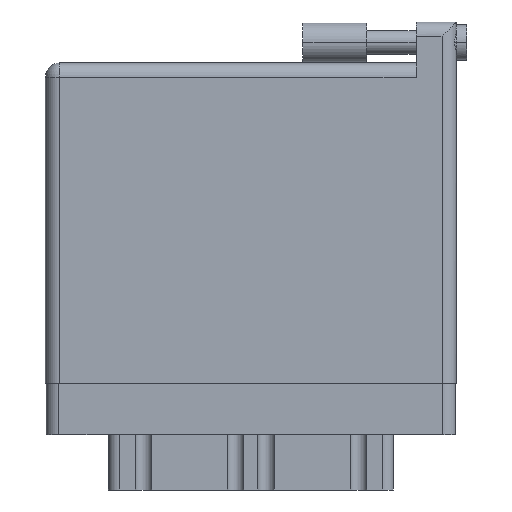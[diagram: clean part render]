
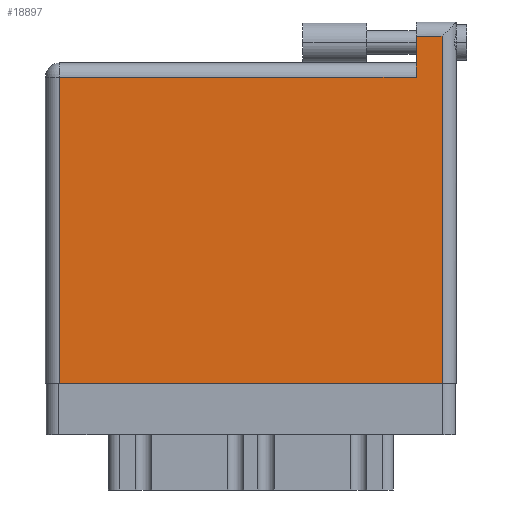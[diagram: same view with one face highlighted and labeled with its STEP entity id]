
A CAD part, front view. The second image highlights one B-rep face of the part: STEP entity #18897.
In plain terms, the highlighted face is planar.
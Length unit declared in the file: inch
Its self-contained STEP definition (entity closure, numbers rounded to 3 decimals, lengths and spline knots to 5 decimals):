
#985 = DIRECTION ( 'NONE',  ( 1., 0., 0. ) ) ;
#2232 = CARTESIAN_POINT ( 'NONE',  ( 0.07, 0., 0. ) ) ;
#2502 = ORIENTED_EDGE ( 'NONE', *, *, #12456, .T. ) ;
#2968 = ORIENTED_EDGE ( 'NONE', *, *, #26892, .T. ) ;
#3290 = FACE_OUTER_BOUND ( 'NONE', #28474, .T. ) ;
#3557 = LINE ( 'NONE', #14199, #27384 ) ;
#4309 = CARTESIAN_POINT ( 'NONE',  ( 0., 1.696, 0. ) ) ;
#5326 = VECTOR ( 'NONE', #9005, 39.37008 ) ;
#5433 = CARTESIAN_POINT ( 'NONE',  ( 1.811, 1.766, 0. ) ) ;
#7760 = VECTOR ( 'NONE', #30245, 39.37008 ) ;
#9005 = DIRECTION ( 'NONE',  ( 0., -1., 0. ) ) ;
#9722 = VECTOR ( 'NONE', #985, 39.37008 ) ;
#9880 = AXIS2_PLACEMENT_3D ( 'NONE', #11156, #13936, #21934 ) ;
#11032 = LINE ( 'NONE', #5433, #19995 ) ;
#11156 = CARTESIAN_POINT ( 'NONE',  ( 0., 1.566, 0. ) ) ;
#11453 = LINE ( 'NONE', #25028, #5326 ) ;
#12249 = VERTEX_POINT ( 'NONE', #2232 ) ;
#12456 = EDGE_CURVE ( 'NONE', #12249, #24019, #30618, .T. ) ;
#12862 = VERTEX_POINT ( 'NONE', #22873 ) ;
#13936 = DIRECTION ( 'NONE',  ( 0., 0., -1. ) ) ;
#14069 = EDGE_CURVE ( 'NONE', #22793, #12862, #11032, .T. ) ;
#14199 = CARTESIAN_POINT ( 'NONE',  ( 1.938, 1.766, 0. ) ) ;
#16367 = ORIENTED_EDGE ( 'NONE', *, *, #14069, .T. ) ;
#17298 = CARTESIAN_POINT ( 'NONE',  ( 0.07, 1.496, 0. ) ) ;
#17603 = EDGE_CURVE ( 'NONE', #21061, #12249, #11453, .T. ) ;
#17937 = CARTESIAN_POINT ( 'NONE',  ( 1.811, 1.696, 0. ) ) ;
#18210 = ORIENTED_EDGE ( 'NONE', *, *, #29429, .T. ) ;
#18897 = ADVANCED_FACE ( 'NONE', ( #3290 ), #29606, .F. ) ;
#19389 = CARTESIAN_POINT ( 'NONE',  ( 1.938, 0., 0. ) ) ;
#19602 = DIRECTION ( 'NONE',  ( 0., 1., 0. ) ) ;
#19995 = VECTOR ( 'NONE', #31580, 39.37008 ) ;
#21061 = VERTEX_POINT ( 'NONE', #17298 ) ;
#21934 = DIRECTION ( 'NONE',  ( -1., 0., 0. ) ) ;
#22793 = VERTEX_POINT ( 'NONE', #17937 ) ;
#22873 = CARTESIAN_POINT ( 'NONE',  ( 1.811, 1.496, 0. ) ) ;
#22993 = VERTEX_POINT ( 'NONE', #27142 ) ;
#24019 = VERTEX_POINT ( 'NONE', #19389 ) ;
#24244 = ORIENTED_EDGE ( 'NONE', *, *, #24831, .T. ) ;
#24831 = EDGE_CURVE ( 'NONE', #12862, #21061, #27969, .T. ) ;
#25028 = CARTESIAN_POINT ( 'NONE',  ( 0.07, 0., 0. ) ) ;
#25183 = CARTESIAN_POINT ( 'NONE',  ( 0., 1.496, 0. ) ) ;
#26892 = EDGE_CURVE ( 'NONE', #24019, #22993, #3557, .T. ) ;
#27142 = CARTESIAN_POINT ( 'NONE',  ( 1.938, 1.696, 0. ) ) ;
#27384 = VECTOR ( 'NONE', #19602, 39.37008 ) ;
#27969 = LINE ( 'NONE', #25183, #7760 ) ;
#28181 = LINE ( 'NONE', #4309, #30870 ) ;
#28474 = EDGE_LOOP ( 'NONE', ( #2502, #2968, #18210, #16367, #24244, #34136 ) ) ;
#29429 = EDGE_CURVE ( 'NONE', #22993, #22793, #28181, .T. ) ;
#29606 = PLANE ( 'NONE',  #9880 ) ;
#30245 = DIRECTION ( 'NONE',  ( -1., 0., 0. ) ) ;
#30442 = CARTESIAN_POINT ( 'NONE',  ( 0., 0., 0. ) ) ;
#30618 = LINE ( 'NONE', #30442, #9722 ) ;
#30870 = VECTOR ( 'NONE', #33572, 39.37008 ) ;
#31580 = DIRECTION ( 'NONE',  ( 0., -1., 0. ) ) ;
#33572 = DIRECTION ( 'NONE',  ( -1., 0., 0. ) ) ;
#34136 = ORIENTED_EDGE ( 'NONE', *, *, #17603, .T. ) ;
